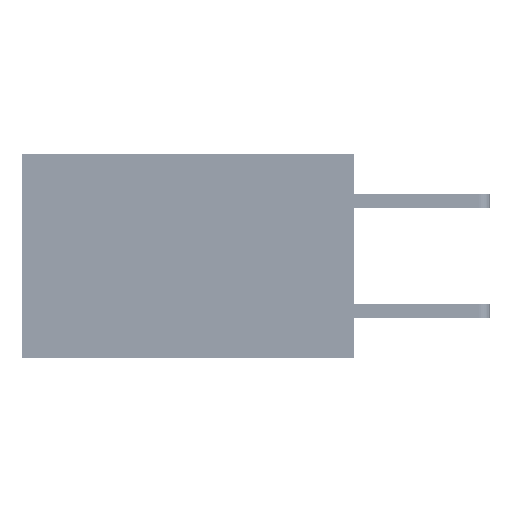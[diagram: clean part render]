
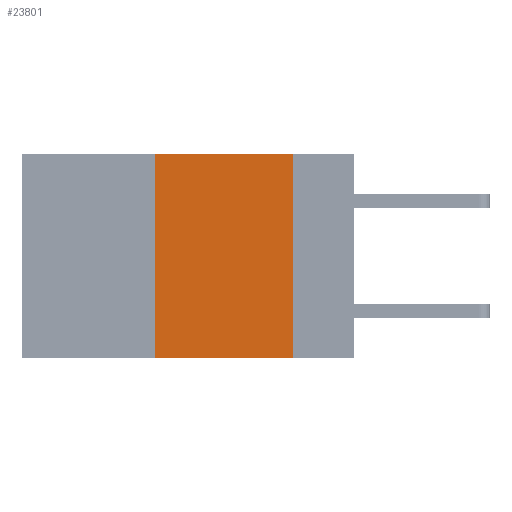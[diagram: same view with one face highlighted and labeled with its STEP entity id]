
A CAD part, left-side view. The second image highlights one B-rep face of the part: STEP entity #23801.
In plain terms, the highlighted planar face has unit normal (-1, 0, 0).
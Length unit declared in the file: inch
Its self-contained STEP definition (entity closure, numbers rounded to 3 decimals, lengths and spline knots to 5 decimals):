
#418 = VERTEX_POINT ( 'NONE', #47592 ) ;
#6397 = EDGE_CURVE ( 'NONE', #418, #47068, #51628, .T. ) ;
#8370 = ORIENTED_EDGE ( 'NONE', *, *, #39680, .F. ) ;
#8400 = EDGE_CURVE ( 'NONE', #47068, #34189, #50830, .T. ) ;
#9003 = PLANE ( 'NONE',  #48685 ) ;
#9922 = ORIENTED_EDGE ( 'NONE', *, *, #6397, .F. ) ;
#12400 = DIRECTION ( 'NONE',  ( 0., -1., 0. ) ) ;
#12914 = CARTESIAN_POINT ( 'NONE',  ( 0., 0.6, -0.37 ) ) ;
#12960 = LINE ( 'NONE', #12914, #27368 ) ;
#13803 = VERTEX_POINT ( 'NONE', #26162 ) ;
#15491 = FACE_OUTER_BOUND ( 'NONE', #41532, .T. ) ;
#16928 = DIRECTION ( 'NONE',  ( 0., -1., 0. ) ) ;
#17754 = ORIENTED_EDGE ( 'NONE', *, *, #45284, .T. ) ;
#21064 = DIRECTION ( 'NONE',  ( 1., 0., 0. ) ) ;
#22536 = CARTESIAN_POINT ( 'NONE',  ( 0., 0.11, -0.37 ) ) ;
#23188 = ORIENTED_EDGE ( 'NONE', *, *, #8400, .F. ) ;
#23801 = ADVANCED_FACE ( 'NONE', ( #15491 ), #9003, .F. ) ;
#26162 = CARTESIAN_POINT ( 'NONE',  ( 0., 0.36, -0.37 ) ) ;
#26931 = CARTESIAN_POINT ( 'NONE',  ( 0., 0.11, 0. ) ) ;
#27368 = VECTOR ( 'NONE', #16928, 39.37008 ) ;
#27447 = CARTESIAN_POINT ( 'NONE',  ( 0., 0.11, 0. ) ) ;
#33134 = DIRECTION ( 'NONE',  ( 0., 0., -1. ) ) ;
#33784 = VECTOR ( 'NONE', #47253, 39.37008 ) ;
#33968 = VECTOR ( 'NONE', #38073, 39.37008 ) ;
#34189 = VERTEX_POINT ( 'NONE', #22536 ) ;
#37893 = CARTESIAN_POINT ( 'NONE',  ( 0., 0.36, 0. ) ) ;
#38073 = DIRECTION ( 'NONE',  ( 0., 0., 1. ) ) ;
#39680 = EDGE_CURVE ( 'NONE', #13803, #418, #40209, .T. ) ;
#40209 = LINE ( 'NONE', #37893, #33968 ) ;
#41479 = VECTOR ( 'NONE', #12400, 39.37008 ) ;
#41532 = EDGE_LOOP ( 'NONE', ( #23188, #9922, #8370, #17754 ) ) ;
#44389 = CARTESIAN_POINT ( 'NONE',  ( 0., 0.6, 0. ) ) ;
#45019 = CARTESIAN_POINT ( 'NONE',  ( 0., 0.6, 0. ) ) ;
#45284 = EDGE_CURVE ( 'NONE', #13803, #34189, #12960, .T. ) ;
#47068 = VERTEX_POINT ( 'NONE', #26931 ) ;
#47253 = DIRECTION ( 'NONE',  ( 0., 0., -1. ) ) ;
#47592 = CARTESIAN_POINT ( 'NONE',  ( 0., 0.36, 0. ) ) ;
#48685 = AXIS2_PLACEMENT_3D ( 'NONE', #45019, #21064, #33134 ) ;
#50830 = LINE ( 'NONE', #27447, #33784 ) ;
#51628 = LINE ( 'NONE', #44389, #41479 ) ;
